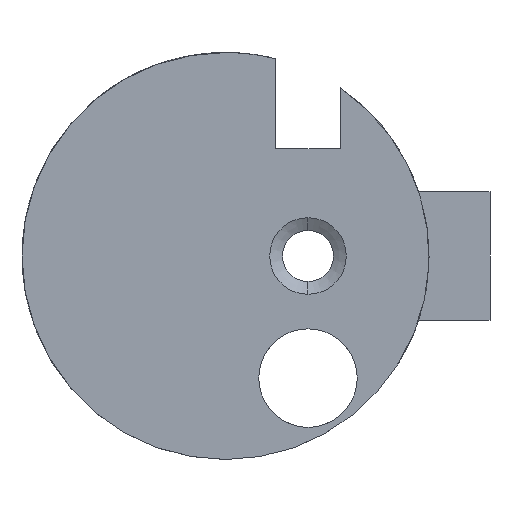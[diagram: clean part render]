
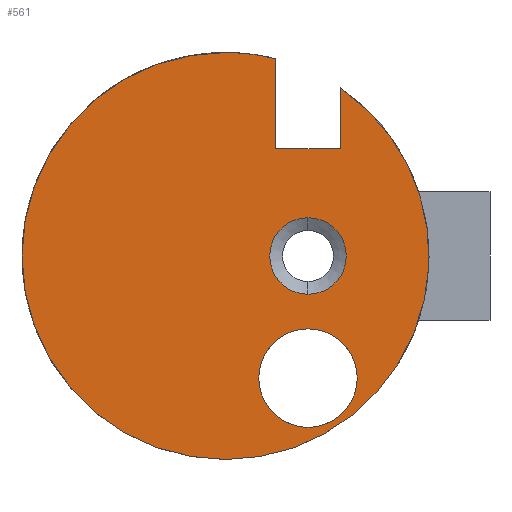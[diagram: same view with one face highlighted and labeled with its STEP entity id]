
A CAD part, left-side view. The second image highlights one B-rep face of the part: STEP entity #561.
In plain terms, the highlighted planar face has unit normal (-1, 0, 0).
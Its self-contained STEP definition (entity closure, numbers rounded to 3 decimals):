
#9 = DIRECTION ( 'NONE',  ( 1., 0., 0. ) ) ;
#16 = ORIENTED_EDGE ( 'NONE', *, *, #1081, .T. ) ;
#22 = FACE_OUTER_BOUND ( 'NONE', #438, .T. ) ;
#26 = CARTESIAN_POINT ( 'NONE',  ( -66.4, 27.397, 5.681 ) ) ;
#29 = ORIENTED_EDGE ( 'NONE', *, *, #43, .F. ) ;
#43 = EDGE_CURVE ( 'NONE', #316, #49, #728, .T. ) ;
#49 = VERTEX_POINT ( 'NONE', #640 ) ;
#53 = CIRCLE ( 'NONE', #917, 9.5 ) ;
#62 = ORIENTED_EDGE ( 'NONE', *, *, #477, .F. ) ;
#72 = DIRECTION ( 'NONE',  ( -1., 0., 0. ) ) ;
#93 = AXIS2_PLACEMENT_3D ( 'NONE', #570, #314, #292 ) ;
#96 = CIRCLE ( 'NONE', #730, 1.786 ) ;
#116 = VERTEX_POINT ( 'NONE', #1092 ) ;
#127 = CARTESIAN_POINT ( 'NONE',  ( -66.4, 27.397, -8.819 ) ) ;
#128 = ORIENTED_EDGE ( 'NONE', *, *, #927, .T. ) ;
#138 = DIRECTION ( 'NONE',  ( 0., 0., 1. ) ) ;
#152 = CIRCLE ( 'NONE', #497, 2.3 ) ;
#197 = DIRECTION ( 'NONE',  ( 1., 0., 0. ) ) ;
#201 = FACE_BOUND ( 'NONE', #300, .T. ) ;
#229 = DIRECTION ( 'NONE',  ( 0., 0., 1. ) ) ;
#238 = ORIENTED_EDGE ( 'NONE', *, *, #650, .T. ) ;
#268 = VERTEX_POINT ( 'NONE', #993 ) ;
#277 = CARTESIAN_POINT ( 'NONE',  ( -66.4, 23.547, -5.019 ) ) ;
#286 = CARTESIAN_POINT ( 'NONE',  ( -66.4, 23.547, -7.319 ) ) ;
#292 = DIRECTION ( 'NONE',  ( 0., 0., 1. ) ) ;
#294 = CARTESIAN_POINT ( 'NONE',  ( -66.4, 27.397, 0.681 ) ) ;
#300 = EDGE_LOOP ( 'NONE', ( #536, #1120 ) ) ;
#303 = CARTESIAN_POINT ( 'NONE',  ( -66.4, 23.547, 2.467 ) ) ;
#314 = DIRECTION ( 'NONE',  ( -1., 0., 0. ) ) ;
#316 = VERTEX_POINT ( 'NONE', #368 ) ;
#328 = EDGE_LOOP ( 'NONE', ( #128, #16 ) ) ;
#349 = VECTOR ( 'NONE', #1097, 1000. ) ;
#360 = CARTESIAN_POINT ( 'NONE',  ( -66.4, 27.397, 10.181 ) ) ;
#361 = CARTESIAN_POINT ( 'NONE',  ( -66.4, 22.047, 8.531 ) ) ;
#368 = CARTESIAN_POINT ( 'NONE',  ( -66.4, 25.047, 9.886 ) ) ;
#391 = FACE_BOUND ( 'NONE', #328, .T. ) ;
#423 = CIRCLE ( 'NONE', #661, 9.5 ) ;
#424 = CIRCLE ( 'NONE', #93, 1.786 ) ;
#428 = VERTEX_POINT ( 'NONE', #303 ) ;
#438 = EDGE_LOOP ( 'NONE', ( #1045, #238, #29, #864, #686, #62 ) ) ;
#477 = EDGE_CURVE ( 'NONE', #1135, #598, #423, .T. ) ;
#494 = EDGE_CURVE ( 'NONE', #598, #977, #583, .T. ) ;
#497 = AXIS2_PLACEMENT_3D ( 'NONE', #277, #741, #1004 ) ;
#536 = ORIENTED_EDGE ( 'NONE', *, *, #998, .F. ) ;
#540 = DIRECTION ( 'NONE',  ( 0., 0., -1. ) ) ;
#560 = LINE ( 'NONE', #26, #1131 ) ;
#561 = ADVANCED_FACE ( 'NONE', ( #201, #391, #22 ), #750, .T. ) ;
#570 = CARTESIAN_POINT ( 'NONE',  ( -66.4, 23.547, 0.681 ) ) ;
#571 = AXIS2_PLACEMENT_3D ( 'NONE', #685, #769, #1055 ) ;
#583 = CIRCLE ( 'NONE', #634, 9.5 ) ;
#588 = CARTESIAN_POINT ( 'NONE',  ( -66.4, 23.547, -5.019 ) ) ;
#598 = VERTEX_POINT ( 'NONE', #127 ) ;
#634 = AXIS2_PLACEMENT_3D ( 'NONE', #763, #9, #1044 ) ;
#636 = CIRCLE ( 'NONE', #762, 2.3 ) ;
#640 = CARTESIAN_POINT ( 'NONE',  ( -66.4, 25.047, 5.681 ) ) ;
#650 = EDGE_CURVE ( 'NONE', #268, #49, #560, .T. ) ;
#661 = AXIS2_PLACEMENT_3D ( 'NONE', #294, #197, #675 ) ;
#675 = DIRECTION ( 'NONE',  ( 0., 0., 1. ) ) ;
#685 = CARTESIAN_POINT ( 'NONE',  ( -66.4, 27.397, 10.181 ) ) ;
#686 = ORIENTED_EDGE ( 'NONE', *, *, #494, .F. ) ;
#693 = VERTEX_POINT ( 'NONE', #1141 ) ;
#708 = EDGE_CURVE ( 'NONE', #116, #428, #424, .T. ) ;
#711 = CARTESIAN_POINT ( 'NONE',  ( -66.4, 27.397, 0.681 ) ) ;
#723 = DIRECTION ( 'NONE',  ( 0., 0., 1. ) ) ;
#728 = LINE ( 'NONE', #1106, #349 ) ;
#730 = AXIS2_PLACEMENT_3D ( 'NONE', #1187, #72, #723 ) ;
#741 = DIRECTION ( 'NONE',  ( 1., 0., 0. ) ) ;
#750 = PLANE ( 'NONE',  #571 ) ;
#762 = AXIS2_PLACEMENT_3D ( 'NONE', #588, #970, #229 ) ;
#763 = CARTESIAN_POINT ( 'NONE',  ( -66.4, 27.397, 0.681 ) ) ;
#769 = DIRECTION ( 'NONE',  ( -1., 0., 0. ) ) ;
#864 = ORIENTED_EDGE ( 'NONE', *, *, #865, .F. ) ;
#865 = EDGE_CURVE ( 'NONE', #977, #316, #53, .T. ) ;
#917 = AXIS2_PLACEMENT_3D ( 'NONE', #711, #1147, #138 ) ;
#926 = DIRECTION ( 'NONE',  ( 0., 1., 0. ) ) ;
#927 = EDGE_CURVE ( 'NONE', #693, #1121, #636, .T. ) ;
#970 = DIRECTION ( 'NONE',  ( 1., 0., 0. ) ) ;
#977 = VERTEX_POINT ( 'NONE', #360 ) ;
#993 = CARTESIAN_POINT ( 'NONE',  ( -66.4, 22.047, 5.681 ) ) ;
#996 = LINE ( 'NONE', #1182, #1017 ) ;
#998 = EDGE_CURVE ( 'NONE', #428, #116, #96, .T. ) ;
#1004 = DIRECTION ( 'NONE',  ( 0., 0., 1. ) ) ;
#1017 = VECTOR ( 'NONE', #540, 1000. ) ;
#1031 = EDGE_CURVE ( 'NONE', #1135, #268, #996, .T. ) ;
#1044 = DIRECTION ( 'NONE',  ( 0., 0., 1. ) ) ;
#1045 = ORIENTED_EDGE ( 'NONE', *, *, #1031, .T. ) ;
#1055 = DIRECTION ( 'NONE',  ( 0., 0., 1. ) ) ;
#1081 = EDGE_CURVE ( 'NONE', #1121, #693, #152, .T. ) ;
#1092 = CARTESIAN_POINT ( 'NONE',  ( -66.4, 23.547, -1.105 ) ) ;
#1097 = DIRECTION ( 'NONE',  ( 0., 0., -1. ) ) ;
#1106 = CARTESIAN_POINT ( 'NONE',  ( -66.4, 25.047, 14.681 ) ) ;
#1120 = ORIENTED_EDGE ( 'NONE', *, *, #708, .F. ) ;
#1121 = VERTEX_POINT ( 'NONE', #286 ) ;
#1131 = VECTOR ( 'NONE', #926, 1000. ) ;
#1135 = VERTEX_POINT ( 'NONE', #361 ) ;
#1141 = CARTESIAN_POINT ( 'NONE',  ( -66.4, 23.547, -2.719 ) ) ;
#1147 = DIRECTION ( 'NONE',  ( 1., 0., 0. ) ) ;
#1182 = CARTESIAN_POINT ( 'NONE',  ( -66.4, 22.047, 10.181 ) ) ;
#1187 = CARTESIAN_POINT ( 'NONE',  ( -66.4, 23.547, 0.681 ) ) ;
